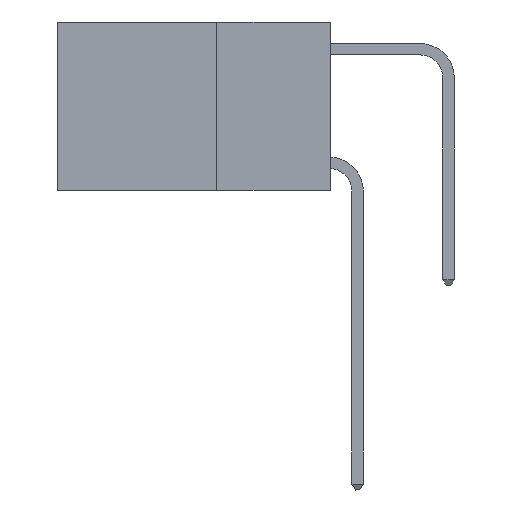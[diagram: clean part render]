
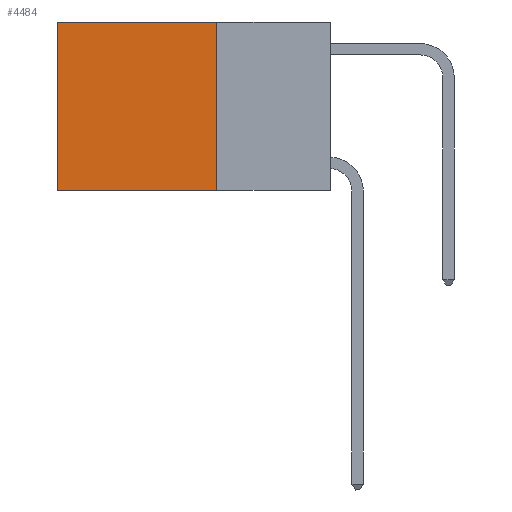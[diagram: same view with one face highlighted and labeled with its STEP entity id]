
A CAD part, left-side view. The second image highlights one B-rep face of the part: STEP entity #4484.
In plain terms, the highlighted planar face has unit normal (-1, 0, 0).
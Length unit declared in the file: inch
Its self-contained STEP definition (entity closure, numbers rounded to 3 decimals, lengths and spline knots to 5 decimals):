
#493 = EDGE_CURVE ( 'NONE', #12152, #10065, #9123, .T. ) ;
#758 = VECTOR ( 'NONE', #2307, 39.37008 ) ;
#1864 = AXIS2_PLACEMENT_3D ( 'NONE', #1890, #8805, #2895 ) ;
#1890 = CARTESIAN_POINT ( 'NONE',  ( 0.2625, 0.25, 0. ) ) ;
#2307 = DIRECTION ( 'NONE',  ( 0., 1., 0. ) ) ;
#2585 = DIRECTION ( 'NONE',  ( 0., 0., -1. ) ) ;
#2730 = CARTESIAN_POINT ( 'NONE',  ( 0.2625, 0.6, -0.37 ) ) ;
#2848 = VERTEX_POINT ( 'NONE', #4129 ) ;
#2895 = DIRECTION ( 'NONE',  ( 0., 0., -1. ) ) ;
#2959 = VECTOR ( 'NONE', #3633, 39.37008 ) ;
#3327 = VECTOR ( 'NONE', #9781, 39.37008 ) ;
#3633 = DIRECTION ( 'NONE',  ( 0., 1., 0. ) ) ;
#3944 = ORIENTED_EDGE ( 'NONE', *, *, #10634, .F. ) ;
#4129 = CARTESIAN_POINT ( 'NONE',  ( 0.2625, 0.25, 0. ) ) ;
#4157 = FACE_OUTER_BOUND ( 'NONE', #9249, .T. ) ;
#4479 = VERTEX_POINT ( 'NONE', #11626 ) ;
#4484 = ADVANCED_FACE ( 'NONE', ( #4157 ), #12542, .F. ) ;
#5895 = CARTESIAN_POINT ( 'NONE',  ( 0.2625, 0.6, 0. ) ) ;
#6245 = LINE ( 'NONE', #5895, #3327 ) ;
#7359 = EDGE_CURVE ( 'NONE', #2848, #4479, #8689, .T. ) ;
#7566 = ORIENTED_EDGE ( 'NONE', *, *, #7359, .T. ) ;
#7877 = LINE ( 'NONE', #8557, #12314 ) ;
#8079 = ORIENTED_EDGE ( 'NONE', *, *, #12522, .T. ) ;
#8254 = CARTESIAN_POINT ( 'NONE',  ( 0.2625, 0.25, -0.37 ) ) ;
#8557 = CARTESIAN_POINT ( 'NONE',  ( 0.2625, 0.25, 0. ) ) ;
#8689 = LINE ( 'NONE', #9193, #758 ) ;
#8805 = DIRECTION ( 'NONE',  ( 1., 0., 0. ) ) ;
#9123 = LINE ( 'NONE', #12310, #2959 ) ;
#9193 = CARTESIAN_POINT ( 'NONE',  ( 0.2625, 0.25, 0. ) ) ;
#9249 = EDGE_LOOP ( 'NONE', ( #8079, #11536, #3944, #7566 ) ) ;
#9781 = DIRECTION ( 'NONE',  ( 0., 0., -1. ) ) ;
#10065 = VERTEX_POINT ( 'NONE', #2730 ) ;
#10634 = EDGE_CURVE ( 'NONE', #2848, #12152, #7877, .T. ) ;
#11536 = ORIENTED_EDGE ( 'NONE', *, *, #493, .F. ) ;
#11626 = CARTESIAN_POINT ( 'NONE',  ( 0.2625, 0.6, 0. ) ) ;
#12152 = VERTEX_POINT ( 'NONE', #8254 ) ;
#12310 = CARTESIAN_POINT ( 'NONE',  ( 0.2625, 0.25, -0.37 ) ) ;
#12314 = VECTOR ( 'NONE', #2585, 39.37008 ) ;
#12522 = EDGE_CURVE ( 'NONE', #4479, #10065, #6245, .T. ) ;
#12542 = PLANE ( 'NONE',  #1864 ) ;
